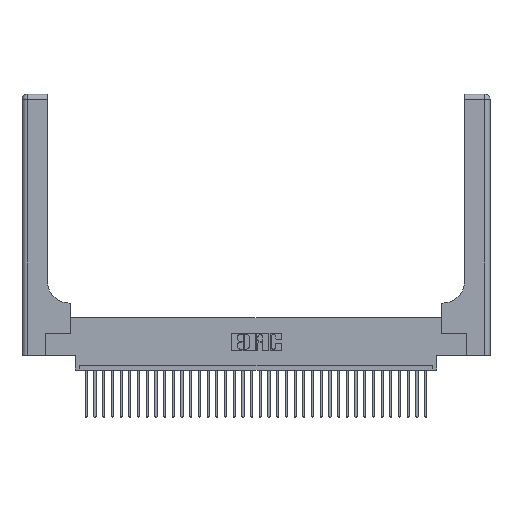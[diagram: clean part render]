
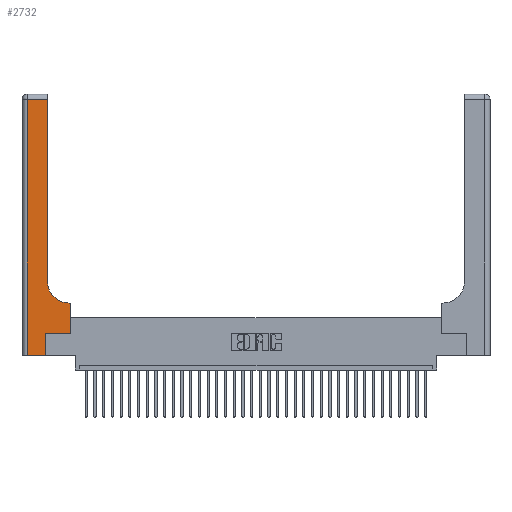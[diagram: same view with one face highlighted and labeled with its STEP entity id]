
A CAD part, top view. The second image highlights one B-rep face of the part: STEP entity #2732.
In plain terms, the highlighted planar face has unit normal (0, 0, 1).
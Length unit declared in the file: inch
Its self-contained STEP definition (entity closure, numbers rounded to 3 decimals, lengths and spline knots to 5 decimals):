
#107 = CARTESIAN_POINT ( 'NONE',  ( 0., 0., 0.37 ) ) ;
#340 = VERTEX_POINT ( 'NONE', #29232 ) ;
#523 = VERTEX_POINT ( 'NONE', #16831 ) ;
#1969 = VERTEX_POINT ( 'NONE', #25791 ) ;
#2032 = CARTESIAN_POINT ( 'NONE',  ( 0.269, 0., 0.37 ) ) ;
#2048 = VERTEX_POINT ( 'NONE', #18528 ) ;
#2258 = CARTESIAN_POINT ( 'NONE',  ( 0.2915, 0.85, 0.37 ) ) ;
#2360 = LINE ( 'NONE', #27212, #22589 ) ;
#2524 = VERTEX_POINT ( 'NONE', #2258 ) ;
#2732 = ADVANCED_FACE ( 'NONE', ( #34460 ), #17725, .F. ) ;
#2753 = VERTEX_POINT ( 'NONE', #23009 ) ;
#2817 = DIRECTION ( 'NONE',  ( 1., 0., 0. ) ) ;
#2980 = AXIS2_PLACEMENT_3D ( 'NONE', #18983, #25292, #2817 ) ;
#3300 = CARTESIAN_POINT ( 'NONE',  ( 0.06, 2.94, 0.37 ) ) ;
#4668 = LINE ( 'NONE', #2032, #33024 ) ;
#5175 = ORIENTED_EDGE ( 'NONE', *, *, #18784, .T. ) ;
#5687 = EDGE_CURVE ( 'NONE', #523, #29535, #26976, .T. ) ;
#5694 = DIRECTION ( 'NONE',  ( 1., 0., 0. ) ) ;
#6004 = VERTEX_POINT ( 'NONE', #32133 ) ;
#6895 = DIRECTION ( 'NONE',  ( 0., 0., -1. ) ) ;
#8539 = AXIS2_PLACEMENT_3D ( 'NONE', #31285, #6895, #9641 ) ;
#9641 = DIRECTION ( 'NONE',  ( -1., 0., 0. ) ) ;
#9889 = CARTESIAN_POINT ( 'NONE',  ( 0.2915, 0.6, 0.37 ) ) ;
#10137 = ORIENTED_EDGE ( 'NONE', *, *, #11883, .T. ) ;
#10605 = LINE ( 'NONE', #10699, #16647 ) ;
#10699 = CARTESIAN_POINT ( 'NONE',  ( 0.2915, 3., 0.37 ) ) ;
#10919 = ORIENTED_EDGE ( 'NONE', *, *, #32837, .T. ) ;
#11070 = CARTESIAN_POINT ( 'NONE',  ( 0.269, 0.25, 0.37 ) ) ;
#11789 = ORIENTED_EDGE ( 'NONE', *, *, #27732, .T. ) ;
#11883 = EDGE_CURVE ( 'NONE', #340, #2753, #18138, .T. ) ;
#12150 = LINE ( 'NONE', #11070, #16048 ) ;
#13464 = CIRCLE ( 'NONE', #2980, 0.25 ) ;
#15495 = EDGE_CURVE ( 'NONE', #6004, #340, #12150, .T. ) ;
#16048 = VECTOR ( 'NONE', #23619, 39.37008 ) ;
#16647 = VECTOR ( 'NONE', #32365, 39.37008 ) ;
#16831 = CARTESIAN_POINT ( 'NONE',  ( 0.2915, 2.94, 0.37 ) ) ;
#17247 = VECTOR ( 'NONE', #22556, 39.37008 ) ;
#17725 = PLANE ( 'NONE',  #8539 ) ;
#18138 = LINE ( 'NONE', #33377, #17247 ) ;
#18528 = CARTESIAN_POINT ( 'NONE',  ( 0.269, 0., 0.37 ) ) ;
#18784 = EDGE_CURVE ( 'NONE', #2524, #523, #10605, .T. ) ;
#18983 = CARTESIAN_POINT ( 'NONE',  ( 0.5415, 0.85, 0.37 ) ) ;
#20084 = CARTESIAN_POINT ( 'NONE',  ( 0., 2.94, 0.37 ) ) ;
#20850 = DIRECTION ( 'NONE',  ( -1., 0., 0. ) ) ;
#22204 = VECTOR ( 'NONE', #5694, 39.37008 ) ;
#22556 = DIRECTION ( 'NONE',  ( 0., 1., 0. ) ) ;
#22589 = VECTOR ( 'NONE', #29470, 39.37008 ) ;
#23009 = CARTESIAN_POINT ( 'NONE',  ( 0.5585, 0.6, 0.37 ) ) ;
#23619 = DIRECTION ( 'NONE',  ( 1., 0., 0. ) ) ;
#23918 = ORIENTED_EDGE ( 'NONE', *, *, #29490, .T. ) ;
#24790 = LINE ( 'NONE', #107, #22204 ) ;
#24909 = CARTESIAN_POINT ( 'NONE',  ( 0.06, 0., 0.37 ) ) ;
#25292 = DIRECTION ( 'NONE',  ( 0., 0., -1. ) ) ;
#25350 = DIRECTION ( 'NONE',  ( -1., 0., 0. ) ) ;
#25729 = EDGE_CURVE ( 'NONE', #2048, #6004, #4668, .T. ) ;
#25791 = CARTESIAN_POINT ( 'NONE',  ( 0.5415, 0.6, 0.37 ) ) ;
#25985 = ORIENTED_EDGE ( 'NONE', *, *, #15495, .T. ) ;
#26976 = LINE ( 'NONE', #20084, #31700 ) ;
#27212 = CARTESIAN_POINT ( 'NONE',  ( 0.06, 3., 0.37 ) ) ;
#27684 = ORIENTED_EDGE ( 'NONE', *, *, #25729, .T. ) ;
#27732 = EDGE_CURVE ( 'NONE', #35125, #2048, #24790, .T. ) ;
#28254 = EDGE_CURVE ( 'NONE', #29535, #35125, #2360, .T. ) ;
#29232 = CARTESIAN_POINT ( 'NONE',  ( 0.5585, 0.25, 0.37 ) ) ;
#29470 = DIRECTION ( 'NONE',  ( 0., -1., 0. ) ) ;
#29490 = EDGE_CURVE ( 'NONE', #1969, #2524, #13464, .T. ) ;
#29535 = VERTEX_POINT ( 'NONE', #3300 ) ;
#30004 = ORIENTED_EDGE ( 'NONE', *, *, #5687, .T. ) ;
#30056 = VECTOR ( 'NONE', #20850, 39.37008 ) ;
#30810 = EDGE_LOOP ( 'NONE', ( #5175, #30004, #33790, #11789, #27684, #25985, #10137, #10919, #23918 ) ) ;
#30926 = LINE ( 'NONE', #9889, #30056 ) ;
#31285 = CARTESIAN_POINT ( 'NONE',  ( 0., 3., 0.37 ) ) ;
#31700 = VECTOR ( 'NONE', #25350, 39.37008 ) ;
#32133 = CARTESIAN_POINT ( 'NONE',  ( 0.269, 0.25, 0.37 ) ) ;
#32365 = DIRECTION ( 'NONE',  ( 0., 1., 0. ) ) ;
#32837 = EDGE_CURVE ( 'NONE', #2753, #1969, #30926, .T. ) ;
#33024 = VECTOR ( 'NONE', #35353, 39.37008 ) ;
#33377 = CARTESIAN_POINT ( 'NONE',  ( 0.5585, 0.25, 0.37 ) ) ;
#33790 = ORIENTED_EDGE ( 'NONE', *, *, #28254, .T. ) ;
#34460 = FACE_OUTER_BOUND ( 'NONE', #30810, .T. ) ;
#35125 = VERTEX_POINT ( 'NONE', #24909 ) ;
#35353 = DIRECTION ( 'NONE',  ( 0., 1., 0. ) ) ;
